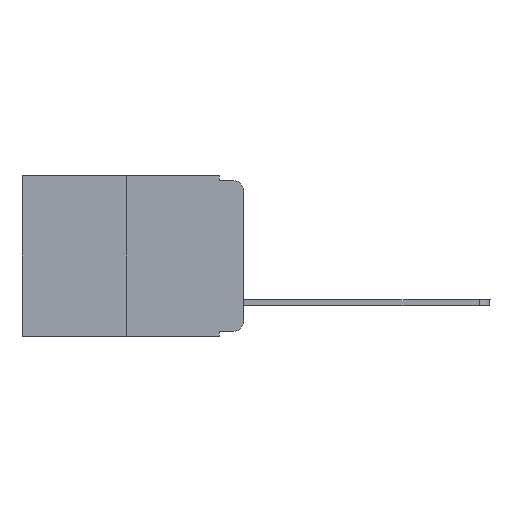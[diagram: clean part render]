
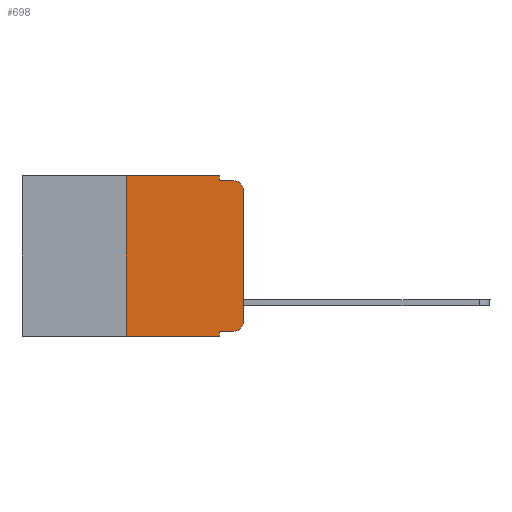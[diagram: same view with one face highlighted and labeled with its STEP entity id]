
A CAD part, left-side view. The second image highlights one B-rep face of the part: STEP entity #698.
In plain terms, the highlighted planar face has unit normal (-1, 0, 0).
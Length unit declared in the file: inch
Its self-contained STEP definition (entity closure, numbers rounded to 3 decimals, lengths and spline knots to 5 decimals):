
#156 = VERTEX_POINT ( 'NONE', #5618 ) ;
#286 = PLANE ( 'NONE',  #7444 ) ;
#478 = DIRECTION ( 'NONE',  ( -1., 0., 0. ) ) ;
#529 = ORIENTED_EDGE ( 'NONE', *, *, #10289, .F. ) ;
#558 = VERTEX_POINT ( 'NONE', #2745 ) ;
#697 = LINE ( 'NONE', #2638, #1447 ) ;
#698 = ADVANCED_FACE ( 'NONE', ( #7938 ), #286, .F. ) ;
#717 = LINE ( 'NONE', #6680, #1877 ) ;
#837 = EDGE_CURVE ( 'NONE', #9072, #5715, #5241, .T. ) ;
#855 = CARTESIAN_POINT ( 'NONE',  ( 0., 0.051, -0.333 ) ) ;
#1005 = CARTESIAN_POINT ( 'NONE',  ( 0., 0.25, 0. ) ) ;
#1221 = DIRECTION ( 'NONE',  ( 1., 0., 0. ) ) ;
#1447 = VECTOR ( 'NONE', #2702, 39.37008 ) ;
#1527 = EDGE_CURVE ( 'NONE', #156, #9072, #717, .T. ) ;
#1537 = CIRCLE ( 'NONE', #11590, 0.02 ) ;
#1717 = VECTOR ( 'NONE', #11445, 39.37008 ) ;
#1877 = VECTOR ( 'NONE', #5508, 39.37008 ) ;
#1957 = ORIENTED_EDGE ( 'NONE', *, *, #8527, .T. ) ;
#2099 = DIRECTION ( 'NONE',  ( 0., 0., -1. ) ) ;
#2138 = LINE ( 'NONE', #3021, #1717 ) ;
#2154 = DIRECTION ( 'NONE',  ( 0., -1., 0. ) ) ;
#2403 = VERTEX_POINT ( 'NONE', #6749 ) ;
#2617 = ORIENTED_EDGE ( 'NONE', *, *, #8798, .F. ) ;
#2638 = CARTESIAN_POINT ( 'NONE',  ( 0., 0.051, 0. ) ) ;
#2702 = DIRECTION ( 'NONE',  ( 0., 0., -1. ) ) ;
#2745 = CARTESIAN_POINT ( 'NONE',  ( 0., 0.051, 0. ) ) ;
#3021 = CARTESIAN_POINT ( 'NONE',  ( 0., 0.051, 0. ) ) ;
#3137 = ORIENTED_EDGE ( 'NONE', *, *, #4310, .F. ) ;
#3139 = DIRECTION ( 'NONE',  ( -1., 0., 0. ) ) ;
#3177 = ORIENTED_EDGE ( 'NONE', *, *, #9654, .T. ) ;
#3420 = CARTESIAN_POINT ( 'NONE',  ( 0., 0.02, -0.03 ) ) ;
#3428 = VERTEX_POINT ( 'NONE', #4972 ) ;
#3625 = DIRECTION ( 'NONE',  ( 0., -1., 0. ) ) ;
#4310 = EDGE_CURVE ( 'NONE', #558, #7740, #2138, .T. ) ;
#4372 = EDGE_CURVE ( 'NONE', #7740, #5715, #9593, .T. ) ;
#4563 = LINE ( 'NONE', #1005, #10275 ) ;
#4917 = VERTEX_POINT ( 'NONE', #6226 ) ;
#4972 = CARTESIAN_POINT ( 'NONE',  ( 0., 0.051, -0.343 ) ) ;
#5058 = EDGE_CURVE ( 'NONE', #6580, #558, #8709, .T. ) ;
#5241 = CIRCLE ( 'NONE', #8394, 0.02 ) ;
#5375 = CARTESIAN_POINT ( 'NONE',  ( 0., 0.02, -0.01 ) ) ;
#5470 = VERTEX_POINT ( 'NONE', #855 ) ;
#5508 = DIRECTION ( 'NONE',  ( 0., 0., 1. ) ) ;
#5618 = CARTESIAN_POINT ( 'NONE',  ( 0., 0., -0.313 ) ) ;
#5675 = ORIENTED_EDGE ( 'NONE', *, *, #10597, .T. ) ;
#5715 = VERTEX_POINT ( 'NONE', #5375 ) ;
#5819 = VECTOR ( 'NONE', #8399, 39.37008 ) ;
#6226 = CARTESIAN_POINT ( 'NONE',  ( 0., 0.02, -0.333 ) ) ;
#6522 = ORIENTED_EDGE ( 'NONE', *, *, #837, .T. ) ;
#6547 = VECTOR ( 'NONE', #2154, 39.37008 ) ;
#6580 = VERTEX_POINT ( 'NONE', #9181 ) ;
#6594 = VECTOR ( 'NONE', #3625, 39.37008 ) ;
#6680 = CARTESIAN_POINT ( 'NONE',  ( 0., 0., 0. ) ) ;
#6749 = CARTESIAN_POINT ( 'NONE',  ( 0., 0.25, -0.343 ) ) ;
#6787 = ORIENTED_EDGE ( 'NONE', *, *, #4372, .F. ) ;
#7008 = CARTESIAN_POINT ( 'NONE',  ( 0., 0.051, -0.01 ) ) ;
#7011 = CARTESIAN_POINT ( 'NONE',  ( 0., 0.473, 0. ) ) ;
#7444 = AXIS2_PLACEMENT_3D ( 'NONE', #7011, #1221, #2099 ) ;
#7641 = LINE ( 'NONE', #9431, #6594 ) ;
#7675 = DIRECTION ( 'NONE',  ( 0., -1., 0. ) ) ;
#7719 = DIRECTION ( 'NONE',  ( 0., 0., -1. ) ) ;
#7740 = VERTEX_POINT ( 'NONE', #7008 ) ;
#7938 = FACE_OUTER_BOUND ( 'NONE', #10934, .T. ) ;
#8146 = ORIENTED_EDGE ( 'NONE', *, *, #5058, .F. ) ;
#8325 = DIRECTION ( 'NONE',  ( 0., 0., 1. ) ) ;
#8394 = AXIS2_PLACEMENT_3D ( 'NONE', #3420, #478, #9012 ) ;
#8399 = DIRECTION ( 'NONE',  ( 0., -1., 0. ) ) ;
#8509 = CARTESIAN_POINT ( 'NONE',  ( 0., 0.473, -0.343 ) ) ;
#8527 = EDGE_CURVE ( 'NONE', #4917, #156, #1537, .T. ) ;
#8692 = CARTESIAN_POINT ( 'NONE',  ( 0., 0.051, -0.01 ) ) ;
#8709 = LINE ( 'NONE', #10660, #6547 ) ;
#8798 = EDGE_CURVE ( 'NONE', #5470, #3428, #697, .T. ) ;
#8865 = CARTESIAN_POINT ( 'NONE',  ( 0., 0.02, -0.313 ) ) ;
#9012 = DIRECTION ( 'NONE',  ( 0., 0., -1. ) ) ;
#9072 = VERTEX_POINT ( 'NONE', #11365 ) ;
#9181 = CARTESIAN_POINT ( 'NONE',  ( 0., 0.25, 0. ) ) ;
#9431 = CARTESIAN_POINT ( 'NONE',  ( 0., 0.051, -0.333 ) ) ;
#9593 = LINE ( 'NONE', #8692, #10564 ) ;
#9654 = EDGE_CURVE ( 'NONE', #2403, #3428, #11382, .T. ) ;
#10275 = VECTOR ( 'NONE', #8325, 39.37008 ) ;
#10289 = EDGE_CURVE ( 'NONE', #2403, #6580, #4563, .T. ) ;
#10490 = ORIENTED_EDGE ( 'NONE', *, *, #1527, .T. ) ;
#10564 = VECTOR ( 'NONE', #7675, 39.37008 ) ;
#10597 = EDGE_CURVE ( 'NONE', #5470, #4917, #7641, .T. ) ;
#10660 = CARTESIAN_POINT ( 'NONE',  ( 0., 0.473, 0. ) ) ;
#10934 = EDGE_LOOP ( 'NONE', ( #10490, #6522, #6787, #3137, #8146, #529, #3177, #2617, #5675, #1957 ) ) ;
#11365 = CARTESIAN_POINT ( 'NONE',  ( 0., 0., -0.03 ) ) ;
#11382 = LINE ( 'NONE', #8509, #5819 ) ;
#11445 = DIRECTION ( 'NONE',  ( 0., 0., -1. ) ) ;
#11590 = AXIS2_PLACEMENT_3D ( 'NONE', #8865, #3139, #7719 ) ;
